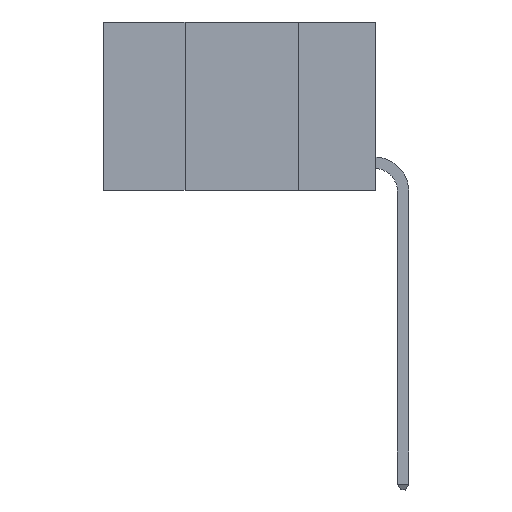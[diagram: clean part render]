
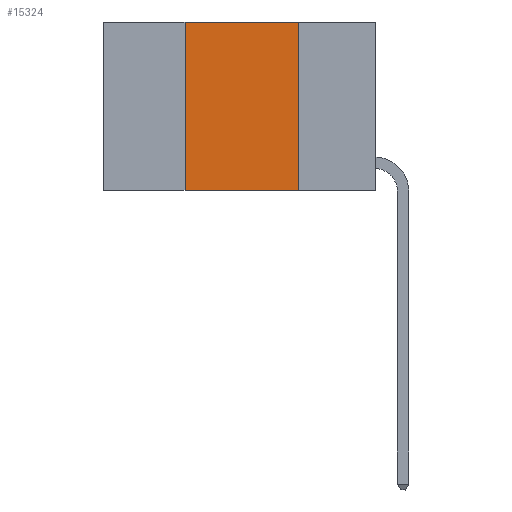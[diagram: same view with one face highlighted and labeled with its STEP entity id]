
A CAD part, left-side view. The second image highlights one B-rep face of the part: STEP entity #15324.
In plain terms, the highlighted planar face has unit normal (-1, 0, 0).
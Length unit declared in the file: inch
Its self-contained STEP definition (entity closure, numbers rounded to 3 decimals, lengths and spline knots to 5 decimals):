
#227 = DIRECTION ( 'NONE',  ( 0., 0., 1. ) ) ;
#555 = ORIENTED_EDGE ( 'NONE', *, *, #9823, .F. ) ;
#720 = ORIENTED_EDGE ( 'NONE', *, *, #747, .F. ) ;
#747 = EDGE_CURVE ( 'NONE', #7347, #5311, #10827, .T. ) ;
#786 = ORIENTED_EDGE ( 'NONE', *, *, #10265, .F. ) ;
#800 = VERTEX_POINT ( 'NONE', #3053 ) ;
#816 = ORIENTED_EDGE ( 'NONE', *, *, #10203, .T. ) ;
#988 = CARTESIAN_POINT ( 'NONE',  ( 0., 0.6, 0. ) ) ;
#1261 = AXIS2_PLACEMENT_3D ( 'NONE', #988, #10530, #2480 ) ;
#1437 = VECTOR ( 'NONE', #227, 39.37008 ) ;
#2480 = DIRECTION ( 'NONE',  ( 0., 0., -1. ) ) ;
#2531 = LINE ( 'NONE', #5778, #15546 ) ;
#2927 = EDGE_LOOP ( 'NONE', ( #555, #720, #786, #816 ) ) ;
#3053 = CARTESIAN_POINT ( 'NONE',  ( 0., 0.42, -0.37 ) ) ;
#3597 = CARTESIAN_POINT ( 'NONE',  ( 0., 0.17, -0.37 ) ) ;
#3600 = LINE ( 'NONE', #12968, #7669 ) ;
#4958 = CARTESIAN_POINT ( 'NONE',  ( 0., 0.6, 0. ) ) ;
#5129 = DIRECTION ( 'NONE',  ( 0., 0., -1. ) ) ;
#5311 = VERTEX_POINT ( 'NONE', #9510 ) ;
#5778 = CARTESIAN_POINT ( 'NONE',  ( 0., 0.6, -0.37 ) ) ;
#5840 = DIRECTION ( 'NONE',  ( 0., -1., 0. ) ) ;
#6962 = VERTEX_POINT ( 'NONE', #3597 ) ;
#7232 = FACE_OUTER_BOUND ( 'NONE', #2927, .T. ) ;
#7347 = VERTEX_POINT ( 'NONE', #15895 ) ;
#7669 = VECTOR ( 'NONE', #5129, 39.37008 ) ;
#8628 = CARTESIAN_POINT ( 'NONE',  ( 0., 0.42, 0. ) ) ;
#9510 = CARTESIAN_POINT ( 'NONE',  ( 0., 0.17, 0. ) ) ;
#9823 = EDGE_CURVE ( 'NONE', #5311, #6962, #3600, .T. ) ;
#10203 = EDGE_CURVE ( 'NONE', #800, #6962, #2531, .T. ) ;
#10265 = EDGE_CURVE ( 'NONE', #800, #7347, #14629, .T. ) ;
#10530 = DIRECTION ( 'NONE',  ( 1., 0., 0. ) ) ;
#10827 = LINE ( 'NONE', #4958, #14171 ) ;
#12968 = CARTESIAN_POINT ( 'NONE',  ( 0., 0.17, 0. ) ) ;
#14171 = VECTOR ( 'NONE', #5840, 39.37008 ) ;
#14629 = LINE ( 'NONE', #8628, #1437 ) ;
#15324 = ADVANCED_FACE ( 'NONE', ( #7232 ), #15455, .F. ) ;
#15455 = PLANE ( 'NONE',  #1261 ) ;
#15546 = VECTOR ( 'NONE', #15959, 39.37008 ) ;
#15895 = CARTESIAN_POINT ( 'NONE',  ( 0., 0.42, 0. ) ) ;
#15959 = DIRECTION ( 'NONE',  ( 0., -1., 0. ) ) ;
